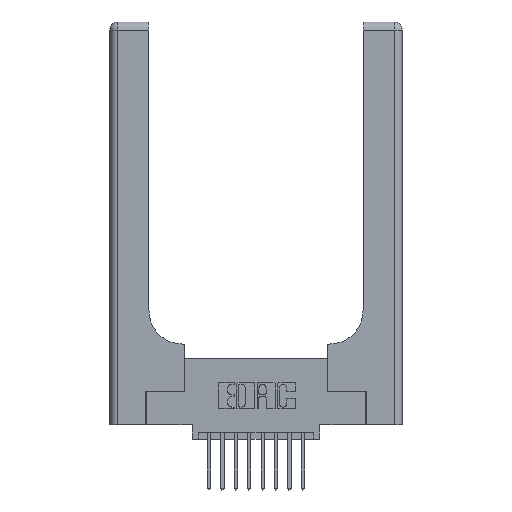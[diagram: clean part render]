
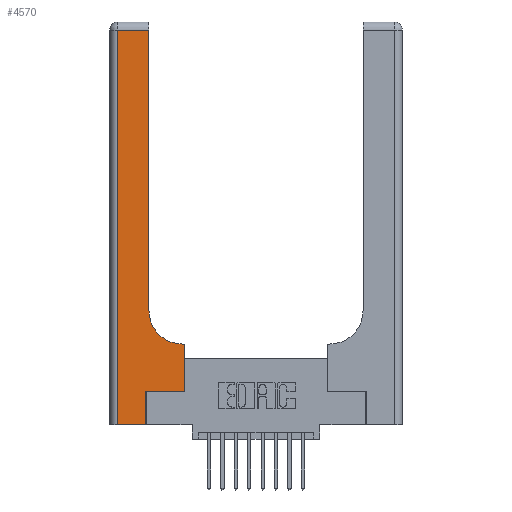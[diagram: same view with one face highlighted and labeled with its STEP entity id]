
A CAD part, top view. The second image highlights one B-rep face of the part: STEP entity #4570.
In plain terms, the highlighted planar face has unit normal (0, 0, 1).
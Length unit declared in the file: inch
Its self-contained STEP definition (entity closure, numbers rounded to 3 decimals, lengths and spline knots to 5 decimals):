
#378 = CARTESIAN_POINT ( 'NONE',  ( 0.06, 2.94, 0.37 ) ) ;
#725 = ORIENTED_EDGE ( 'NONE', *, *, #4114, .T. ) ;
#858 = CARTESIAN_POINT ( 'NONE',  ( 0.269, 0.25, 0.37 ) ) ;
#912 = VECTOR ( 'NONE', #13031, 39.37008 ) ;
#1053 = VECTOR ( 'NONE', #1388, 39.37008 ) ;
#1168 = CARTESIAN_POINT ( 'NONE',  ( 0.06, 3., 0.37 ) ) ;
#1176 = VECTOR ( 'NONE', #13872, 39.37008 ) ;
#1388 = DIRECTION ( 'NONE',  ( 0., -1., 0. ) ) ;
#1402 = VECTOR ( 'NONE', #12114, 39.37008 ) ;
#1630 = CARTESIAN_POINT ( 'NONE',  ( 0.2915, 3., 0.37 ) ) ;
#1825 = EDGE_CURVE ( 'NONE', #4935, #5128, #8247, .T. ) ;
#1872 = EDGE_CURVE ( 'NONE', #3435, #11711, #10416, .T. ) ;
#2173 = CIRCLE ( 'NONE', #9054, 0.25 ) ;
#2224 = CARTESIAN_POINT ( 'NONE',  ( 0.06, 0., 0.37 ) ) ;
#2762 = CARTESIAN_POINT ( 'NONE',  ( 0.2915, 0.85, 0.37 ) ) ;
#3435 = VERTEX_POINT ( 'NONE', #6180 ) ;
#3651 = VECTOR ( 'NONE', #10685, 39.37008 ) ;
#3802 = EDGE_CURVE ( 'NONE', #5128, #6726, #4749, .T. ) ;
#3886 = ORIENTED_EDGE ( 'NONE', *, *, #15321, .T. ) ;
#4114 = EDGE_CURVE ( 'NONE', #9639, #4935, #4169, .T. ) ;
#4169 = LINE ( 'NONE', #1630, #10896 ) ;
#4196 = CARTESIAN_POINT ( 'NONE',  ( 0.2915, 0.6, 0.37 ) ) ;
#4491 = DIRECTION ( 'NONE',  ( 0., 0., -1. ) ) ;
#4570 = ADVANCED_FACE ( 'NONE', ( #10522 ), #7801, .F. ) ;
#4749 = LINE ( 'NONE', #1168, #1053 ) ;
#4866 = LINE ( 'NONE', #7575, #1176 ) ;
#4935 = VERTEX_POINT ( 'NONE', #14971 ) ;
#5023 = CARTESIAN_POINT ( 'NONE',  ( 0., 0., 0.37 ) ) ;
#5128 = VERTEX_POINT ( 'NONE', #378 ) ;
#5416 = ORIENTED_EDGE ( 'NONE', *, *, #6933, .T. ) ;
#5596 = ORIENTED_EDGE ( 'NONE', *, *, #1825, .T. ) ;
#6180 = CARTESIAN_POINT ( 'NONE',  ( 0.269, 0., 0.37 ) ) ;
#6237 = EDGE_LOOP ( 'NONE', ( #725, #5596, #10627, #5416, #10808, #15245, #3886, #14683, #14877 ) ) ;
#6726 = VERTEX_POINT ( 'NONE', #2224 ) ;
#6825 = CARTESIAN_POINT ( 'NONE',  ( 0.269, 0.25, 0.37 ) ) ;
#6851 = VECTOR ( 'NONE', #11402, 39.37008 ) ;
#6933 = EDGE_CURVE ( 'NONE', #6726, #3435, #13942, .T. ) ;
#7135 = CARTESIAN_POINT ( 'NONE',  ( 0.269, 0., 0.37 ) ) ;
#7444 = VECTOR ( 'NONE', #14347, 39.37008 ) ;
#7520 = VERTEX_POINT ( 'NONE', #7679 ) ;
#7575 = CARTESIAN_POINT ( 'NONE',  ( 0.5585, 0.25, 0.37 ) ) ;
#7599 = CARTESIAN_POINT ( 'NONE',  ( 0.5415, 0.6, 0.37 ) ) ;
#7679 = CARTESIAN_POINT ( 'NONE',  ( 0.5585, 0.25, 0.37 ) ) ;
#7801 = PLANE ( 'NONE',  #11814 ) ;
#7952 = EDGE_CURVE ( 'NONE', #9617, #10097, #13507, .T. ) ;
#8247 = LINE ( 'NONE', #15672, #7444 ) ;
#8524 = LINE ( 'NONE', #858, #1402 ) ;
#9054 = AXIS2_PLACEMENT_3D ( 'NONE', #12045, #4491, #13319 ) ;
#9617 = VERTEX_POINT ( 'NONE', #11495 ) ;
#9639 = VERTEX_POINT ( 'NONE', #2762 ) ;
#10097 = VERTEX_POINT ( 'NONE', #7599 ) ;
#10416 = LINE ( 'NONE', #7135, #3651 ) ;
#10522 = FACE_OUTER_BOUND ( 'NONE', #6237, .T. ) ;
#10627 = ORIENTED_EDGE ( 'NONE', *, *, #3802, .T. ) ;
#10685 = DIRECTION ( 'NONE',  ( 0., 1., 0. ) ) ;
#10808 = ORIENTED_EDGE ( 'NONE', *, *, #1872, .T. ) ;
#10896 = VECTOR ( 'NONE', #15492, 39.37008 ) ;
#11402 = DIRECTION ( 'NONE',  ( 1., 0., 0. ) ) ;
#11495 = CARTESIAN_POINT ( 'NONE',  ( 0.5585, 0.6, 0.37 ) ) ;
#11711 = VERTEX_POINT ( 'NONE', #6825 ) ;
#11814 = AXIS2_PLACEMENT_3D ( 'NONE', #12111, #11871, #11854 ) ;
#11854 = DIRECTION ( 'NONE',  ( -1., 0., 0. ) ) ;
#11871 = DIRECTION ( 'NONE',  ( 0., 0., -1. ) ) ;
#12045 = CARTESIAN_POINT ( 'NONE',  ( 0.5415, 0.85, 0.37 ) ) ;
#12111 = CARTESIAN_POINT ( 'NONE',  ( 0., 3., 0.37 ) ) ;
#12114 = DIRECTION ( 'NONE',  ( 1., 0., 0. ) ) ;
#12384 = EDGE_CURVE ( 'NONE', #11711, #7520, #8524, .T. ) ;
#13031 = DIRECTION ( 'NONE',  ( -1., 0., 0. ) ) ;
#13319 = DIRECTION ( 'NONE',  ( 1., 0., 0. ) ) ;
#13507 = LINE ( 'NONE', #4196, #912 ) ;
#13872 = DIRECTION ( 'NONE',  ( 0., 1., 0. ) ) ;
#13942 = LINE ( 'NONE', #5023, #6851 ) ;
#14347 = DIRECTION ( 'NONE',  ( -1., 0., 0. ) ) ;
#14683 = ORIENTED_EDGE ( 'NONE', *, *, #7952, .T. ) ;
#14877 = ORIENTED_EDGE ( 'NONE', *, *, #15030, .T. ) ;
#14971 = CARTESIAN_POINT ( 'NONE',  ( 0.2915, 2.94, 0.37 ) ) ;
#15030 = EDGE_CURVE ( 'NONE', #10097, #9639, #2173, .T. ) ;
#15245 = ORIENTED_EDGE ( 'NONE', *, *, #12384, .T. ) ;
#15321 = EDGE_CURVE ( 'NONE', #7520, #9617, #4866, .T. ) ;
#15492 = DIRECTION ( 'NONE',  ( 0., 1., 0. ) ) ;
#15672 = CARTESIAN_POINT ( 'NONE',  ( 0., 2.94, 0.37 ) ) ;
